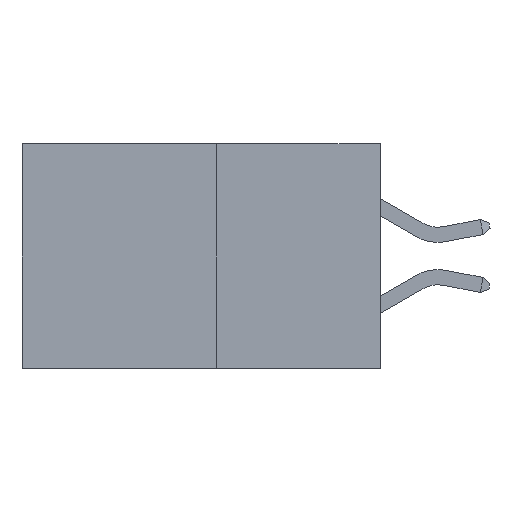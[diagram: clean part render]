
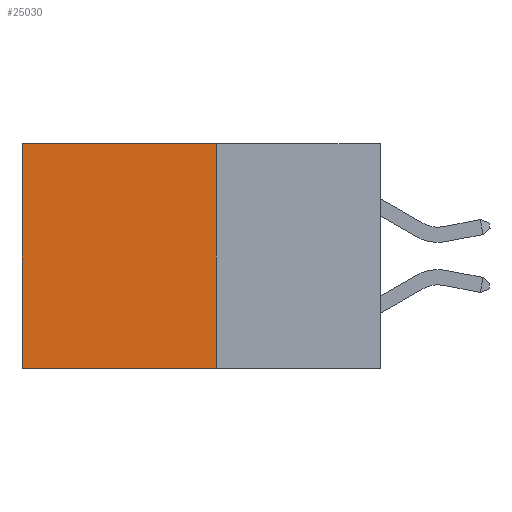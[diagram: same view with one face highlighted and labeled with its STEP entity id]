
A CAD part, left-side view. The second image highlights one B-rep face of the part: STEP entity #25030.
In plain terms, the highlighted planar face has unit normal (-1, 0, 0).
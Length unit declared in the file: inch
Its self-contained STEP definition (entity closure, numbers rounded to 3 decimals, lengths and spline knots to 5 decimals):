
#1193 = CARTESIAN_POINT ( 'NONE',  ( 0.277, 0.27, 0. ) ) ;
#4177 = CARTESIAN_POINT ( 'NONE',  ( 0.277, 0.27, -0.37 ) ) ;
#4518 = VECTOR ( 'NONE', #26317, 39.37008 ) ;
#5189 = VECTOR ( 'NONE', #16801, 39.37008 ) ;
#5421 = VECTOR ( 'NONE', #19918, 39.37008 ) ;
#5427 = CARTESIAN_POINT ( 'NONE',  ( 0.277, 0.27, -0.37 ) ) ;
#5665 = ORIENTED_EDGE ( 'NONE', *, *, #9708, .F. ) ;
#7005 = LINE ( 'NONE', #32428, #5421 ) ;
#9128 = DIRECTION ( 'NONE',  ( 0., 0., -1. ) ) ;
#9708 = EDGE_CURVE ( 'NONE', #23915, #32679, #17185, .T. ) ;
#10448 = AXIS2_PLACEMENT_3D ( 'NONE', #19664, #32282, #17212 ) ;
#10659 = VECTOR ( 'NONE', #9128, 39.37008 ) ;
#11231 = CARTESIAN_POINT ( 'NONE',  ( 0.277, 0.27, -0.37 ) ) ;
#13273 = EDGE_CURVE ( 'NONE', #15330, #32679, #16586, .T. ) ;
#14669 = PLANE ( 'NONE',  #10448 ) ;
#15330 = VERTEX_POINT ( 'NONE', #27096 ) ;
#16586 = LINE ( 'NONE', #24235, #10659 ) ;
#16801 = DIRECTION ( 'NONE',  ( 0., 0., -1. ) ) ;
#17185 = LINE ( 'NONE', #11231, #4518 ) ;
#17212 = DIRECTION ( 'NONE',  ( 0., 0., -1. ) ) ;
#17308 = EDGE_LOOP ( 'NONE', ( #23679, #5665, #20737, #32496 ) ) ;
#17875 = VERTEX_POINT ( 'NONE', #1193 ) ;
#19664 = CARTESIAN_POINT ( 'NONE',  ( 0.277, 0.27, -0.37 ) ) ;
#19918 = DIRECTION ( 'NONE',  ( 0., 1., 0. ) ) ;
#20299 = CARTESIAN_POINT ( 'NONE',  ( 0.277, 0.59, -0.37 ) ) ;
#20737 = ORIENTED_EDGE ( 'NONE', *, *, #22164, .F. ) ;
#22164 = EDGE_CURVE ( 'NONE', #17875, #23915, #31226, .T. ) ;
#23679 = ORIENTED_EDGE ( 'NONE', *, *, #13273, .T. ) ;
#23915 = VERTEX_POINT ( 'NONE', #5427 ) ;
#24235 = CARTESIAN_POINT ( 'NONE',  ( 0.277, 0.59, -0.37 ) ) ;
#25030 = ADVANCED_FACE ( 'NONE', ( #31876 ), #14669, .F. ) ;
#26317 = DIRECTION ( 'NONE',  ( 0., 1., 0. ) ) ;
#27096 = CARTESIAN_POINT ( 'NONE',  ( 0.277, 0.59, 0. ) ) ;
#29791 = EDGE_CURVE ( 'NONE', #17875, #15330, #7005, .T. ) ;
#31226 = LINE ( 'NONE', #4177, #5189 ) ;
#31876 = FACE_OUTER_BOUND ( 'NONE', #17308, .T. ) ;
#32282 = DIRECTION ( 'NONE',  ( 1., 0., 0. ) ) ;
#32428 = CARTESIAN_POINT ( 'NONE',  ( 0.277, 0.27, 0. ) ) ;
#32496 = ORIENTED_EDGE ( 'NONE', *, *, #29791, .T. ) ;
#32679 = VERTEX_POINT ( 'NONE', #20299 ) ;
